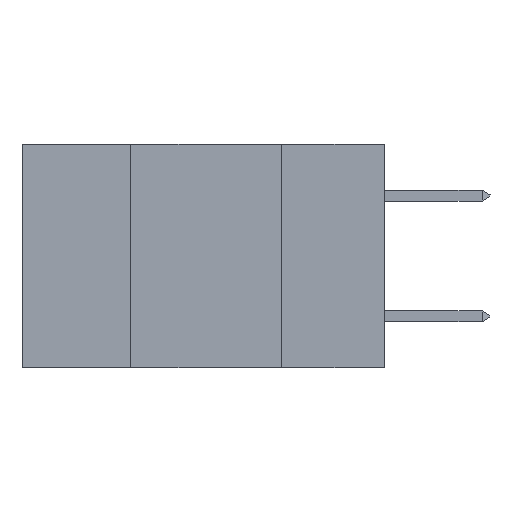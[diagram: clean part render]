
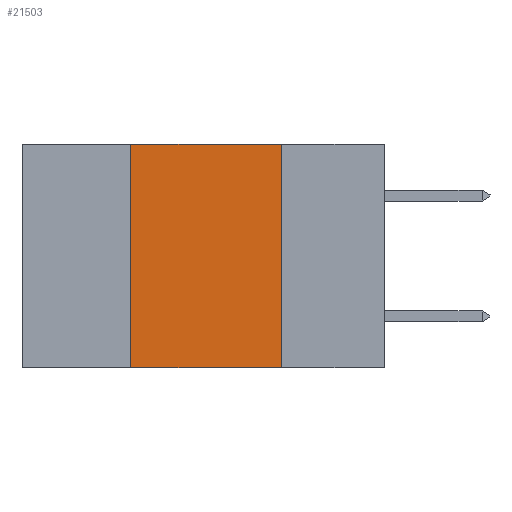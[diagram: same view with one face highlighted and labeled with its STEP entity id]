
A CAD part, left-side view. The second image highlights one B-rep face of the part: STEP entity #21503.
In plain terms, the highlighted planar face has unit normal (-1, 0, 0).
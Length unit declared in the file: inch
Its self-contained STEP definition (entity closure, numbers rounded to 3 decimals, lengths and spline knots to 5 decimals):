
#283 = CARTESIAN_POINT ( 'NONE',  ( 0., 0.17, -0.37 ) ) ;
#286 = VERTEX_POINT ( 'NONE', #24011 ) ;
#1670 = LINE ( 'NONE', #16321, #22872 ) ;
#1881 = CARTESIAN_POINT ( 'NONE',  ( 0., 0.17, 0. ) ) ;
#3645 = DIRECTION ( 'NONE',  ( 0., -1., 0. ) ) ;
#6118 = VECTOR ( 'NONE', #10446, 39.37008 ) ;
#7477 = CARTESIAN_POINT ( 'NONE',  ( 0., 0.6, 0. ) ) ;
#7716 = VERTEX_POINT ( 'NONE', #283 ) ;
#8298 = DIRECTION ( 'NONE',  ( 0., -1., 0. ) ) ;
#9060 = ORIENTED_EDGE ( 'NONE', *, *, #12752, .T. ) ;
#9062 = CARTESIAN_POINT ( 'NONE',  ( 0., 0.17, 0. ) ) ;
#9586 = DIRECTION ( 'NONE',  ( 0., 0., -1. ) ) ;
#10440 = DIRECTION ( 'NONE',  ( 0., 0., 1. ) ) ;
#10446 = DIRECTION ( 'NONE',  ( 0., 0., -1. ) ) ;
#10862 = VECTOR ( 'NONE', #10440, 39.37008 ) ;
#10880 = EDGE_CURVE ( 'NONE', #286, #18306, #20304, .T. ) ;
#11531 = LINE ( 'NONE', #12449, #10862 ) ;
#12033 = ORIENTED_EDGE ( 'NONE', *, *, #23151, .F. ) ;
#12449 = CARTESIAN_POINT ( 'NONE',  ( 0., 0.42, 0. ) ) ;
#12752 = EDGE_CURVE ( 'NONE', #16181, #7716, #1670, .T. ) ;
#13345 = ORIENTED_EDGE ( 'NONE', *, *, #10880, .F. ) ;
#14814 = FACE_OUTER_BOUND ( 'NONE', #24377, .T. ) ;
#16181 = VERTEX_POINT ( 'NONE', #22197 ) ;
#16321 = CARTESIAN_POINT ( 'NONE',  ( 0., 0.6, -0.37 ) ) ;
#17338 = LINE ( 'NONE', #1881, #6118 ) ;
#18306 = VERTEX_POINT ( 'NONE', #9062 ) ;
#20127 = PLANE ( 'NONE',  #25354 ) ;
#20304 = LINE ( 'NONE', #20947, #25210 ) ;
#20947 = CARTESIAN_POINT ( 'NONE',  ( 0., 0.6, 0. ) ) ;
#21229 = EDGE_CURVE ( 'NONE', #16181, #286, #11531, .T. ) ;
#21503 = ADVANCED_FACE ( 'NONE', ( #14814 ), #20127, .F. ) ;
#22197 = CARTESIAN_POINT ( 'NONE',  ( 0., 0.42, -0.37 ) ) ;
#22240 = DIRECTION ( 'NONE',  ( 1., 0., 0. ) ) ;
#22872 = VECTOR ( 'NONE', #3645, 39.37008 ) ;
#23151 = EDGE_CURVE ( 'NONE', #18306, #7716, #17338, .T. ) ;
#23256 = ORIENTED_EDGE ( 'NONE', *, *, #21229, .F. ) ;
#24011 = CARTESIAN_POINT ( 'NONE',  ( 0., 0.42, 0. ) ) ;
#24377 = EDGE_LOOP ( 'NONE', ( #12033, #13345, #23256, #9060 ) ) ;
#25210 = VECTOR ( 'NONE', #8298, 39.37008 ) ;
#25354 = AXIS2_PLACEMENT_3D ( 'NONE', #7477, #22240, #9586 ) ;
